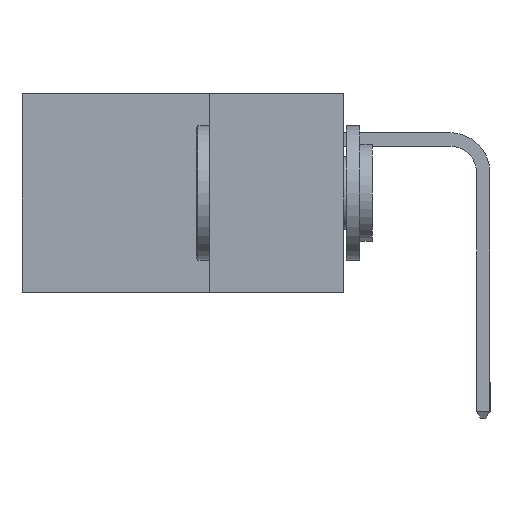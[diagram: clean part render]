
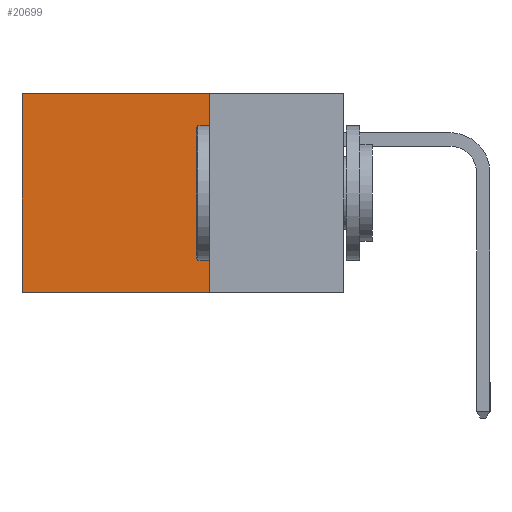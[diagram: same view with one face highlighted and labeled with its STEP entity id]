
A CAD part, left-side view. The second image highlights one B-rep face of the part: STEP entity #20699.
In plain terms, the highlighted planar face has unit normal (-1, 0, 0).
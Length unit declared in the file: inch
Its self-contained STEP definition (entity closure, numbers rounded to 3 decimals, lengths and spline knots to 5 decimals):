
#2186 = VERTEX_POINT ( 'NONE', #12449 ) ;
#2791 = VECTOR ( 'NONE', #3877, 39.37008 ) ;
#2881 = VECTOR ( 'NONE', #3276, 39.37008 ) ;
#2928 = DIRECTION ( 'NONE',  ( 0., 0., -1. ) ) ;
#3276 = DIRECTION ( 'NONE',  ( 0., 1., 0. ) ) ;
#3877 = DIRECTION ( 'NONE',  ( 0., 0., -1. ) ) ;
#4146 = CARTESIAN_POINT ( 'NONE',  ( 0.298, 0.25, -0.37 ) ) ;
#4269 = EDGE_CURVE ( 'NONE', #18276, #21796, #21911, .T. ) ;
#4801 = ORIENTED_EDGE ( 'NONE', *, *, #4269, .T. ) ;
#4894 = CARTESIAN_POINT ( 'NONE',  ( 0.298, 0.25, 0. ) ) ;
#6448 = CARTESIAN_POINT ( 'NONE',  ( 0.298, 0.6, 0. ) ) ;
#6540 = AXIS2_PLACEMENT_3D ( 'NONE', #8849, #22064, #10771 ) ;
#7605 = CARTESIAN_POINT ( 'NONE',  ( 0.298, 0.25, 0. ) ) ;
#8578 = VECTOR ( 'NONE', #2928, 39.37008 ) ;
#8849 = CARTESIAN_POINT ( 'NONE',  ( 0.298, 0.25, 0. ) ) ;
#9136 = EDGE_CURVE ( 'NONE', #18276, #2186, #23659, .T. ) ;
#9176 = VECTOR ( 'NONE', #11854, 39.37008 ) ;
#10771 = DIRECTION ( 'NONE',  ( 0., 0., -1. ) ) ;
#11854 = DIRECTION ( 'NONE',  ( 0., 1., 0. ) ) ;
#12449 = CARTESIAN_POINT ( 'NONE',  ( 0.298, 0.25, -0.37 ) ) ;
#17007 = FACE_OUTER_BOUND ( 'NONE', #24198, .T. ) ;
#17357 = EDGE_CURVE ( 'NONE', #21796, #23174, #23012, .T. ) ;
#17701 = CARTESIAN_POINT ( 'NONE',  ( 0.298, 0.6, 0. ) ) ;
#18109 = ORIENTED_EDGE ( 'NONE', *, *, #9136, .F. ) ;
#18276 = VERTEX_POINT ( 'NONE', #7605 ) ;
#20161 = PLANE ( 'NONE',  #6540 ) ;
#20699 = ADVANCED_FACE ( 'NONE', ( #17007 ), #20161, .F. ) ;
#20701 = ORIENTED_EDGE ( 'NONE', *, *, #17357, .T. ) ;
#21039 = ORIENTED_EDGE ( 'NONE', *, *, #24187, .F. ) ;
#21796 = VERTEX_POINT ( 'NONE', #6448 ) ;
#21911 = LINE ( 'NONE', #24194, #2881 ) ;
#22064 = DIRECTION ( 'NONE',  ( 1., 0., 0. ) ) ;
#22106 = CARTESIAN_POINT ( 'NONE',  ( 0.298, 0.6, -0.37 ) ) ;
#23012 = LINE ( 'NONE', #17701, #2791 ) ;
#23174 = VERTEX_POINT ( 'NONE', #22106 ) ;
#23659 = LINE ( 'NONE', #4894, #8578 ) ;
#24187 = EDGE_CURVE ( 'NONE', #2186, #23174, #24238, .T. ) ;
#24194 = CARTESIAN_POINT ( 'NONE',  ( 0.298, 0.25, 0. ) ) ;
#24198 = EDGE_LOOP ( 'NONE', ( #20701, #21039, #18109, #4801 ) ) ;
#24238 = LINE ( 'NONE', #4146, #9176 ) ;
